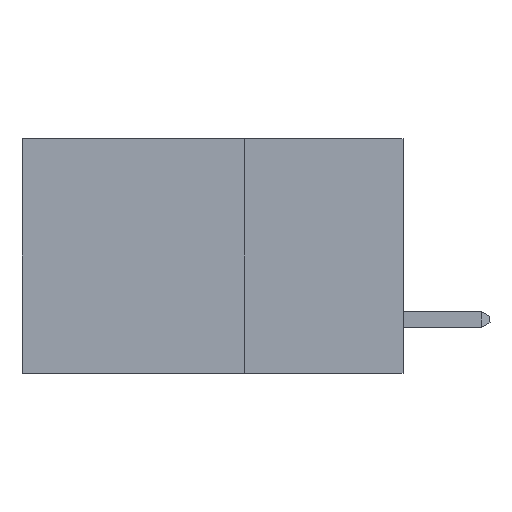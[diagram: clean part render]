
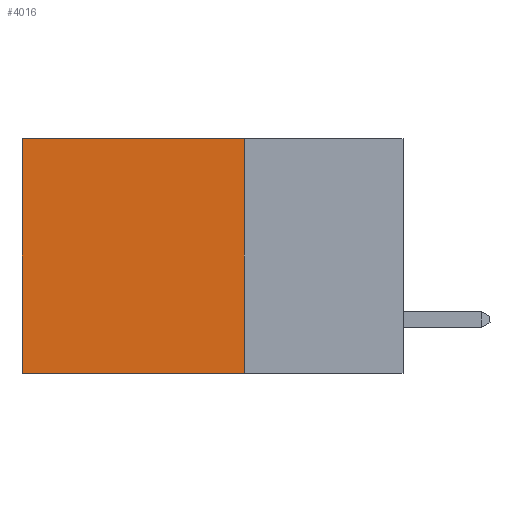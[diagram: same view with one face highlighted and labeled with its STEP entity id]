
A CAD part, left-side view. The second image highlights one B-rep face of the part: STEP entity #4016.
In plain terms, the highlighted planar face has unit normal (-1, 0, 0).
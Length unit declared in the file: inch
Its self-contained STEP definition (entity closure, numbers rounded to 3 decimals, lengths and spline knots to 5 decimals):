
#329 = EDGE_CURVE ( 'NONE', #8731, #6802, #9369, .T. ) ;
#347 = VECTOR ( 'NONE', #6145, 39.37008 ) ;
#369 = CARTESIAN_POINT ( 'NONE',  ( 0.2875, 0.25, -0.37 ) ) ;
#810 = PLANE ( 'NONE',  #1474 ) ;
#835 = DIRECTION ( 'NONE',  ( 1., 0., 0. ) ) ;
#863 = CARTESIAN_POINT ( 'NONE',  ( 0.2875, 0.25, 0. ) ) ;
#1474 = AXIS2_PLACEMENT_3D ( 'NONE', #863, #835, #1783 ) ;
#1783 = DIRECTION ( 'NONE',  ( 0., 0., -1. ) ) ;
#1849 = VERTEX_POINT ( 'NONE', #5814 ) ;
#1964 = CARTESIAN_POINT ( 'NONE',  ( 0.2875, 0.25, -0.37 ) ) ;
#2048 = EDGE_CURVE ( 'NONE', #8731, #4763, #5362, .T. ) ;
#2199 = EDGE_CURVE ( 'NONE', #4763, #1849, #8168, .T. ) ;
#2962 = ORIENTED_EDGE ( 'NONE', *, *, #2199, .T. ) ;
#3003 = DIRECTION ( 'NONE',  ( 0., 1., 0. ) ) ;
#3164 = CARTESIAN_POINT ( 'NONE',  ( 0.2875, 0.6, 0. ) ) ;
#3458 = CARTESIAN_POINT ( 'NONE',  ( 0.2875, 0.25, 0. ) ) ;
#3956 = DIRECTION ( 'NONE',  ( 0., 1., 0. ) ) ;
#4016 = ADVANCED_FACE ( 'NONE', ( #9319 ), #810, .F. ) ;
#4763 = VERTEX_POINT ( 'NONE', #7872 ) ;
#5152 = VECTOR ( 'NONE', #3956, 39.37008 ) ;
#5170 = ORIENTED_EDGE ( 'NONE', *, *, #2048, .T. ) ;
#5362 = LINE ( 'NONE', #8985, #5152 ) ;
#5370 = VECTOR ( 'NONE', #3003, 39.37008 ) ;
#5814 = CARTESIAN_POINT ( 'NONE',  ( 0.2875, 0.6, -0.37 ) ) ;
#6145 = DIRECTION ( 'NONE',  ( 0., 0., -1. ) ) ;
#6802 = VERTEX_POINT ( 'NONE', #1964 ) ;
#7124 = LINE ( 'NONE', #369, #5370 ) ;
#7560 = DIRECTION ( 'NONE',  ( 0., 0., -1. ) ) ;
#7697 = VECTOR ( 'NONE', #7560, 39.37008 ) ;
#7712 = CARTESIAN_POINT ( 'NONE',  ( 0.2875, 0.25, 0. ) ) ;
#7872 = CARTESIAN_POINT ( 'NONE',  ( 0.2875, 0.6, 0. ) ) ;
#8015 = ORIENTED_EDGE ( 'NONE', *, *, #8100, .F. ) ;
#8100 = EDGE_CURVE ( 'NONE', #6802, #1849, #7124, .T. ) ;
#8168 = LINE ( 'NONE', #3164, #347 ) ;
#8327 = EDGE_LOOP ( 'NONE', ( #2962, #8015, #8399, #5170 ) ) ;
#8399 = ORIENTED_EDGE ( 'NONE', *, *, #329, .F. ) ;
#8731 = VERTEX_POINT ( 'NONE', #7712 ) ;
#8985 = CARTESIAN_POINT ( 'NONE',  ( 0.2875, 0.25, 0. ) ) ;
#9319 = FACE_OUTER_BOUND ( 'NONE', #8327, .T. ) ;
#9369 = LINE ( 'NONE', #3458, #7697 ) ;
